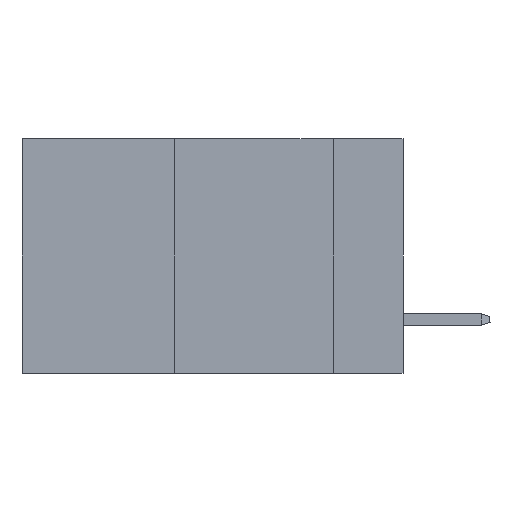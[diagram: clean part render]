
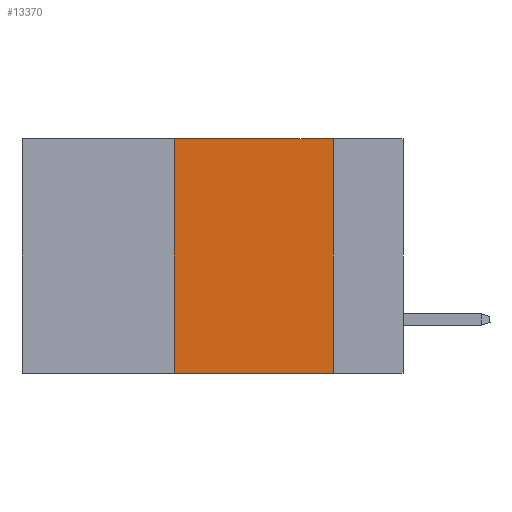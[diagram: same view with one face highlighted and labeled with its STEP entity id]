
A CAD part, left-side view. The second image highlights one B-rep face of the part: STEP entity #13370.
In plain terms, the highlighted planar face has unit normal (-1, 0, 0).
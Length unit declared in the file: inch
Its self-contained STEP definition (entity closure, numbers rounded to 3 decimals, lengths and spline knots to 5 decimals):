
#849 = VECTOR ( 'NONE', #13467, 39.37008 ) ;
#1317 = EDGE_CURVE ( 'NONE', #21548, #10212, #7172, .T. ) ;
#3147 = AXIS2_PLACEMENT_3D ( 'NONE', #9267, #15397, #25872 ) ;
#4107 = EDGE_CURVE ( 'NONE', #14614, #10212, #25900, .T. ) ;
#5431 = DIRECTION ( 'NONE',  ( 0., 0., 1. ) ) ;
#5711 = CARTESIAN_POINT ( 'NONE',  ( 0., 0.11, 0. ) ) ;
#7172 = LINE ( 'NONE', #23797, #13760 ) ;
#7474 = CARTESIAN_POINT ( 'NONE',  ( 0., 0.36, 0. ) ) ;
#7503 = DIRECTION ( 'NONE',  ( 0., -1., 0. ) ) ;
#9267 = CARTESIAN_POINT ( 'NONE',  ( 0., 0.6, 0. ) ) ;
#9531 = PLANE ( 'NONE',  #3147 ) ;
#10082 = CARTESIAN_POINT ( 'NONE',  ( 0., 0.36, -0.37 ) ) ;
#10212 = VERTEX_POINT ( 'NONE', #13199 ) ;
#10444 = ORIENTED_EDGE ( 'NONE', *, *, #13398, .F. ) ;
#10766 = EDGE_CURVE ( 'NONE', #26683, #21548, #19345, .T. ) ;
#13199 = CARTESIAN_POINT ( 'NONE',  ( 0., 0.11, -0.37 ) ) ;
#13370 = ADVANCED_FACE ( 'NONE', ( #15532 ), #9531, .F. ) ;
#13398 = EDGE_CURVE ( 'NONE', #14614, #26683, #17851, .T. ) ;
#13452 = DIRECTION ( 'NONE',  ( 0., 0., -1. ) ) ;
#13467 = DIRECTION ( 'NONE',  ( 0., -1., 0. ) ) ;
#13760 = VECTOR ( 'NONE', #13452, 39.37008 ) ;
#14375 = CARTESIAN_POINT ( 'NONE',  ( 0., 0.36, 0. ) ) ;
#14439 = VECTOR ( 'NONE', #5431, 39.37008 ) ;
#14614 = VERTEX_POINT ( 'NONE', #10082 ) ;
#15397 = DIRECTION ( 'NONE',  ( 1., 0., 0. ) ) ;
#15532 = FACE_OUTER_BOUND ( 'NONE', #19300, .T. ) ;
#17851 = LINE ( 'NONE', #7474, #14439 ) ;
#19190 = ORIENTED_EDGE ( 'NONE', *, *, #10766, .F. ) ;
#19290 = ORIENTED_EDGE ( 'NONE', *, *, #1317, .F. ) ;
#19300 = EDGE_LOOP ( 'NONE', ( #19290, #19190, #10444, #25721 ) ) ;
#19345 = LINE ( 'NONE', #23958, #849 ) ;
#20178 = CARTESIAN_POINT ( 'NONE',  ( 0., 0.6, -0.37 ) ) ;
#21548 = VERTEX_POINT ( 'NONE', #5711 ) ;
#23797 = CARTESIAN_POINT ( 'NONE',  ( 0., 0.11, 0. ) ) ;
#23958 = CARTESIAN_POINT ( 'NONE',  ( 0., 0.6, 0. ) ) ;
#24310 = VECTOR ( 'NONE', #7503, 39.37008 ) ;
#25721 = ORIENTED_EDGE ( 'NONE', *, *, #4107, .T. ) ;
#25872 = DIRECTION ( 'NONE',  ( 0., 0., -1. ) ) ;
#25900 = LINE ( 'NONE', #20178, #24310 ) ;
#26683 = VERTEX_POINT ( 'NONE', #14375 ) ;
